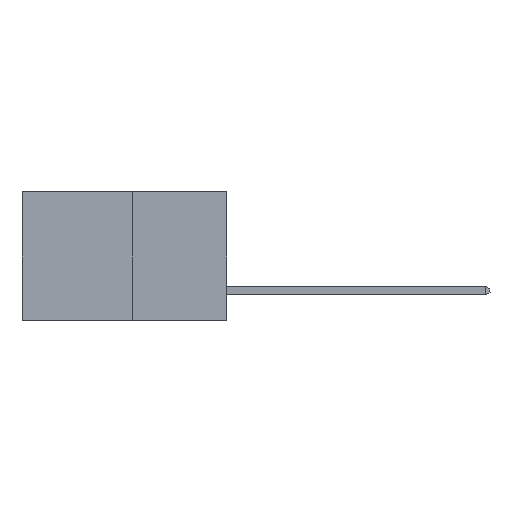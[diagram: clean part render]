
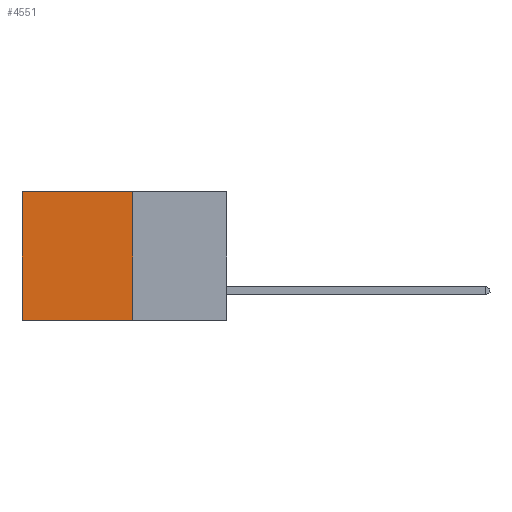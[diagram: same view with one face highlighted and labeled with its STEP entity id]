
A CAD part, left-side view. The second image highlights one B-rep face of the part: STEP entity #4551.
In plain terms, the highlighted planar face has unit normal (-1, 0, 0).
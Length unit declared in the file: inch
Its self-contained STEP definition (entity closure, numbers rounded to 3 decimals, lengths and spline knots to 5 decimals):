
#104 = ORIENTED_EDGE ( 'NONE', *, *, #3433, .F. ) ;
#257 = VERTEX_POINT ( 'NONE', #1667 ) ;
#595 = CARTESIAN_POINT ( 'NONE',  ( 0.277, 0.59, -0.37 ) ) ;
#596 = ORIENTED_EDGE ( 'NONE', *, *, #1759, .F. ) ;
#824 = CARTESIAN_POINT ( 'NONE',  ( 0.277, 0.27, -0.37 ) ) ;
#835 = EDGE_CURVE ( 'NONE', #3036, #5665, #9447, .T. ) ;
#1034 = VECTOR ( 'NONE', #1576, 39.37008 ) ;
#1249 = ORIENTED_EDGE ( 'NONE', *, *, #835, .T. ) ;
#1576 = DIRECTION ( 'NONE',  ( 0., 0., -1. ) ) ;
#1667 = CARTESIAN_POINT ( 'NONE',  ( 0.277, 0.59, -0.37 ) ) ;
#1759 = EDGE_CURVE ( 'NONE', #3036, #2782, #9561, .T. ) ;
#2113 = PLANE ( 'NONE',  #9421 ) ;
#2203 = DIRECTION ( 'NONE',  ( 0., 1., 0. ) ) ;
#2379 = VECTOR ( 'NONE', #5550, 39.37008 ) ;
#2782 = VERTEX_POINT ( 'NONE', #824 ) ;
#2915 = CARTESIAN_POINT ( 'NONE',  ( 0.277, 0.27, 0. ) ) ;
#3036 = VERTEX_POINT ( 'NONE', #2915 ) ;
#3167 = LINE ( 'NONE', #595, #1034 ) ;
#3433 = EDGE_CURVE ( 'NONE', #2782, #257, #4158, .T. ) ;
#3482 = VECTOR ( 'NONE', #7705, 39.37008 ) ;
#3811 = CARTESIAN_POINT ( 'NONE',  ( 0.277, 0.27, 0. ) ) ;
#4158 = LINE ( 'NONE', #6991, #2379 ) ;
#4191 = EDGE_LOOP ( 'NONE', ( #8240, #104, #596, #1249 ) ) ;
#4551 = ADVANCED_FACE ( 'NONE', ( #5832 ), #2113, .F. ) ;
#5329 = VECTOR ( 'NONE', #2203, 39.37008 ) ;
#5354 = CARTESIAN_POINT ( 'NONE',  ( 0.277, 0.59, 0. ) ) ;
#5550 = DIRECTION ( 'NONE',  ( 0., 1., 0. ) ) ;
#5665 = VERTEX_POINT ( 'NONE', #5354 ) ;
#5832 = FACE_OUTER_BOUND ( 'NONE', #4191, .T. ) ;
#5857 = CARTESIAN_POINT ( 'NONE',  ( 0.277, 0.27, -0.37 ) ) ;
#6352 = EDGE_CURVE ( 'NONE', #5665, #257, #3167, .T. ) ;
#6991 = CARTESIAN_POINT ( 'NONE',  ( 0.277, 0.27, -0.37 ) ) ;
#7310 = DIRECTION ( 'NONE',  ( 0., 0., -1. ) ) ;
#7468 = DIRECTION ( 'NONE',  ( 1., 0., 0. ) ) ;
#7705 = DIRECTION ( 'NONE',  ( 0., 0., -1. ) ) ;
#8240 = ORIENTED_EDGE ( 'NONE', *, *, #6352, .T. ) ;
#8449 = CARTESIAN_POINT ( 'NONE',  ( 0.277, 0.27, -0.37 ) ) ;
#9421 = AXIS2_PLACEMENT_3D ( 'NONE', #5857, #7468, #7310 ) ;
#9447 = LINE ( 'NONE', #3811, #5329 ) ;
#9561 = LINE ( 'NONE', #8449, #3482 ) ;
